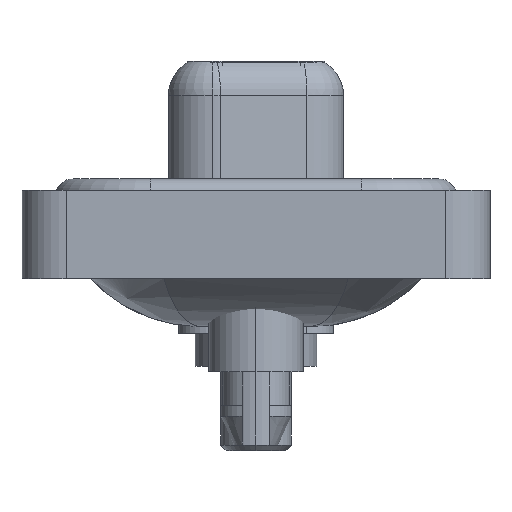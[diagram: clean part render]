
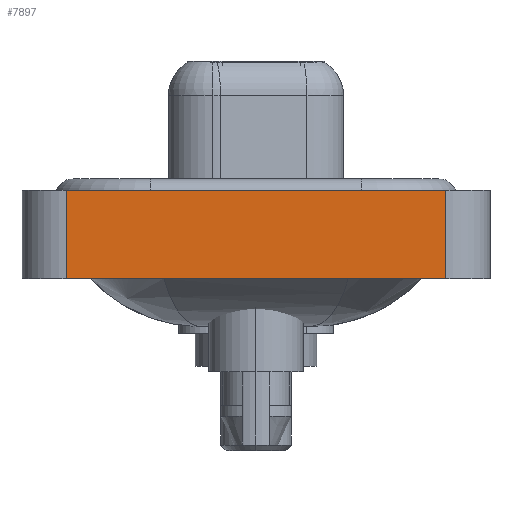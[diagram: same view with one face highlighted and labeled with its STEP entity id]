
A CAD part, left-side view. The second image highlights one B-rep face of the part: STEP entity #7897.
In plain terms, the highlighted planar face has unit normal (-1, 0, 0).
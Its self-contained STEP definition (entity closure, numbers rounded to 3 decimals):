
#490 = CARTESIAN_POINT ( 'NONE',  ( -7.3, -8.55, 0.4 ) ) ;
#1731 = CARTESIAN_POINT ( 'NONE',  ( -7.3, -8.55, -3.6 ) ) ;
#2049 = EDGE_LOOP ( 'NONE', ( #9719, #17179, #4996, #13767 ) ) ;
#2199 = CARTESIAN_POINT ( 'NONE',  ( -7.3, -8.55, -3.6 ) ) ;
#2381 = PLANE ( 'NONE',  #6507 ) ;
#3486 = DIRECTION ( 'NONE',  ( 0., -1., 0. ) ) ;
#3812 = DIRECTION ( 'NONE',  ( -1., 0., 0. ) ) ;
#4068 = EDGE_CURVE ( 'NONE', #10146, #15084, #10233, .T. ) ;
#4298 = VECTOR ( 'NONE', #3486, 1000. ) ;
#4896 = DIRECTION ( 'NONE',  ( 0., -1., 0. ) ) ;
#4975 = DIRECTION ( 'NONE',  ( 0., 0., 1. ) ) ;
#4996 = ORIENTED_EDGE ( 'NONE', *, *, #12707, .F. ) ;
#6507 = AXIS2_PLACEMENT_3D ( 'NONE', #2199, #3812, #4975 ) ;
#7897 = ADVANCED_FACE ( 'NONE', ( #13156 ), #2381, .T. ) ;
#8139 = CARTESIAN_POINT ( 'NONE',  ( -7.3, 8.55, 0.4 ) ) ;
#8245 = CARTESIAN_POINT ( 'NONE',  ( -7.3, 8.55, -3.6 ) ) ;
#8474 = LINE ( 'NONE', #9908, #14067 ) ;
#8482 = VERTEX_POINT ( 'NONE', #8139 ) ;
#9719 = ORIENTED_EDGE ( 'NONE', *, *, #15863, .T. ) ;
#9908 = CARTESIAN_POINT ( 'NONE',  ( -7.3, 8.55, -3.6 ) ) ;
#10146 = VERTEX_POINT ( 'NONE', #8245 ) ;
#10233 = LINE ( 'NONE', #13185, #4298 ) ;
#10995 = LINE ( 'NONE', #16578, #13486 ) ;
#12707 = EDGE_CURVE ( 'NONE', #10146, #8482, #8474, .T. ) ;
#13156 = FACE_OUTER_BOUND ( 'NONE', #2049, .T. ) ;
#13185 = CARTESIAN_POINT ( 'NONE',  ( -7.3, -8.55, -3.6 ) ) ;
#13486 = VECTOR ( 'NONE', #16404, 1000. ) ;
#13767 = ORIENTED_EDGE ( 'NONE', *, *, #4068, .T. ) ;
#14067 = VECTOR ( 'NONE', #15229, 1000. ) ;
#14588 = CARTESIAN_POINT ( 'NONE',  ( -7.3, -8.55, 0.4 ) ) ;
#14773 = EDGE_CURVE ( 'NONE', #8482, #15062, #17060, .T. ) ;
#15062 = VERTEX_POINT ( 'NONE', #490 ) ;
#15084 = VERTEX_POINT ( 'NONE', #1731 ) ;
#15229 = DIRECTION ( 'NONE',  ( 0., 0., 1. ) ) ;
#15863 = EDGE_CURVE ( 'NONE', #15084, #15062, #10995, .T. ) ;
#16404 = DIRECTION ( 'NONE',  ( 0., 0., 1. ) ) ;
#16525 = VECTOR ( 'NONE', #4896, 1000. ) ;
#16578 = CARTESIAN_POINT ( 'NONE',  ( -7.3, -8.55, -3.6 ) ) ;
#17060 = LINE ( 'NONE', #14588, #16525 ) ;
#17179 = ORIENTED_EDGE ( 'NONE', *, *, #14773, .F. ) ;
